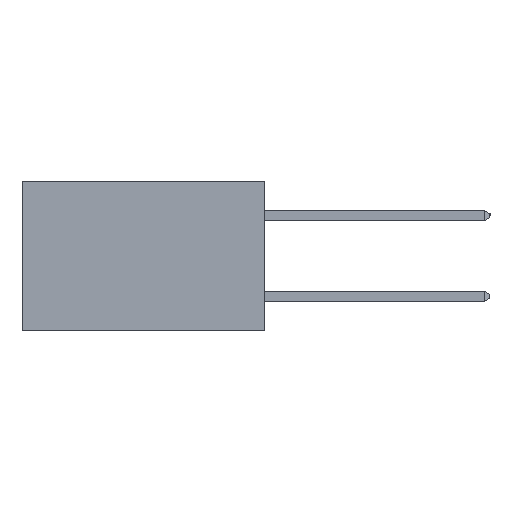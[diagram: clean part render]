
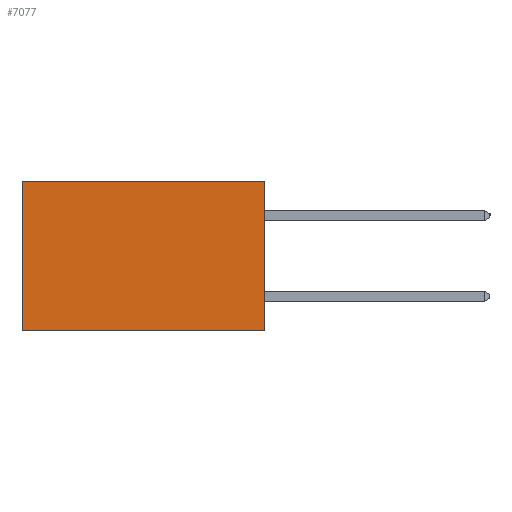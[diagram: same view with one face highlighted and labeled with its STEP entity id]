
A CAD part, left-side view. The second image highlights one B-rep face of the part: STEP entity #7077.
In plain terms, the highlighted planar face has unit normal (-1, 0, 0).
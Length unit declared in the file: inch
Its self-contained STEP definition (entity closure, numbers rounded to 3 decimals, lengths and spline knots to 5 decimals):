
#310 = CARTESIAN_POINT ( 'NONE',  ( 0.298, 0., 0. ) ) ;
#1638 = VECTOR ( 'NONE', #17399, 39.37008 ) ;
#1875 = CARTESIAN_POINT ( 'NONE',  ( 0.298, 0.6, -0.37 ) ) ;
#3322 = CARTESIAN_POINT ( 'NONE',  ( 0.298, 0., 0. ) ) ;
#3353 = VECTOR ( 'NONE', #11220, 39.37008 ) ;
#3666 = ORIENTED_EDGE ( 'NONE', *, *, #7800, .T. ) ;
#3823 = LINE ( 'NONE', #11306, #3353 ) ;
#6133 = LINE ( 'NONE', #17300, #1638 ) ;
#6353 = DIRECTION ( 'NONE',  ( 1., 0., 0. ) ) ;
#6617 = ORIENTED_EDGE ( 'NONE', *, *, #13497, .F. ) ;
#7077 = ADVANCED_FACE ( 'NONE', ( #14521 ), #8040, .F. ) ;
#7264 = VERTEX_POINT ( 'NONE', #3322 ) ;
#7372 = CARTESIAN_POINT ( 'NONE',  ( 0.298, 0., -0.37 ) ) ;
#7711 = DIRECTION ( 'NONE',  ( 0., 0., -1. ) ) ;
#7781 = EDGE_LOOP ( 'NONE', ( #13114, #18067, #6617, #3666 ) ) ;
#7800 = EDGE_CURVE ( 'NONE', #7264, #11693, #17603, .T. ) ;
#8040 = PLANE ( 'NONE',  #12534 ) ;
#8687 = VECTOR ( 'NONE', #14868, 39.37008 ) ;
#9124 = LINE ( 'NONE', #310, #8687 ) ;
#9416 = CARTESIAN_POINT ( 'NONE',  ( 0.298, 0., 0. ) ) ;
#9583 = VECTOR ( 'NONE', #14673, 39.37008 ) ;
#9777 = EDGE_CURVE ( 'NONE', #11693, #15602, #3823, .T. ) ;
#10984 = EDGE_CURVE ( 'NONE', #13293, #15602, #6133, .T. ) ;
#11220 = DIRECTION ( 'NONE',  ( 0., 0., -1. ) ) ;
#11306 = CARTESIAN_POINT ( 'NONE',  ( 0.298, 0.6, 0. ) ) ;
#11693 = VERTEX_POINT ( 'NONE', #11760 ) ;
#11760 = CARTESIAN_POINT ( 'NONE',  ( 0.298, 0.6, 0. ) ) ;
#12534 = AXIS2_PLACEMENT_3D ( 'NONE', #9416, #6353, #7711 ) ;
#13114 = ORIENTED_EDGE ( 'NONE', *, *, #9777, .T. ) ;
#13293 = VERTEX_POINT ( 'NONE', #7372 ) ;
#13497 = EDGE_CURVE ( 'NONE', #7264, #13293, #9124, .T. ) ;
#14521 = FACE_OUTER_BOUND ( 'NONE', #7781, .T. ) ;
#14637 = CARTESIAN_POINT ( 'NONE',  ( 0.298, 0., 0. ) ) ;
#14673 = DIRECTION ( 'NONE',  ( 0., 1., 0. ) ) ;
#14868 = DIRECTION ( 'NONE',  ( 0., 0., -1. ) ) ;
#15602 = VERTEX_POINT ( 'NONE', #1875 ) ;
#17300 = CARTESIAN_POINT ( 'NONE',  ( 0.298, 0., -0.37 ) ) ;
#17399 = DIRECTION ( 'NONE',  ( 0., 1., 0. ) ) ;
#17603 = LINE ( 'NONE', #14637, #9583 ) ;
#18067 = ORIENTED_EDGE ( 'NONE', *, *, #10984, .F. ) ;
